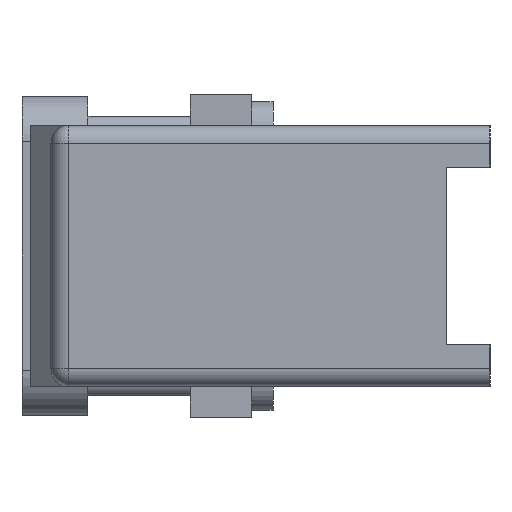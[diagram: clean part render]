
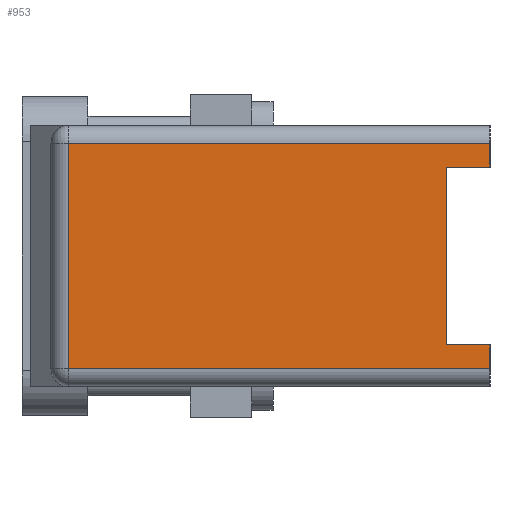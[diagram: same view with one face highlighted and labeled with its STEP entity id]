
A CAD part, left-side view. The second image highlights one B-rep face of the part: STEP entity #953.
In plain terms, the highlighted planar face has unit normal (-1, 0, 0).
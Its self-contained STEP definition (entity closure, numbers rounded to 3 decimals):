
#18 = CARTESIAN_POINT ( 'NONE',  ( 0., 3.81, -3.683 ) ) ;
#96 = CARTESIAN_POINT ( 'NONE',  ( 0., 0., -23.114 ) ) ;
#129 = CARTESIAN_POINT ( 'NONE',  ( 0., 0., -23.114 ) ) ;
#130 = VERTEX_POINT ( 'NONE', #845 ) ;
#219 = LINE ( 'NONE', #2686, #951 ) ;
#231 = LINE ( 'NONE', #2186, #2647 ) ;
#274 = LINE ( 'NONE', #713, #1966 ) ;
#310 = CARTESIAN_POINT ( 'NONE',  ( 0., 0., -23.114 ) ) ;
#330 = PLANE ( 'NONE',  #2122 ) ;
#363 = LINE ( 'NONE', #793, #1813 ) ;
#399 = EDGE_CURVE ( 'NONE', #551, #640, #274, .T. ) ;
#498 = VECTOR ( 'NONE', #2099, 1000. ) ;
#499 = VERTEX_POINT ( 'NONE', #770 ) ;
#533 = VECTOR ( 'NONE', #1638, 1000. ) ;
#551 = VERTEX_POINT ( 'NONE', #1040 ) ;
#559 = CARTESIAN_POINT ( 'NONE',  ( 0., 37.287, -23.114 ) ) ;
#625 = VERTEX_POINT ( 'NONE', #829 ) ;
#640 = VERTEX_POINT ( 'NONE', #1927 ) ;
#713 = CARTESIAN_POINT ( 'NONE',  ( 0., 3.81, -19.431 ) ) ;
#728 = VECTOR ( 'NONE', #2731, 1000. ) ;
#748 = VECTOR ( 'NONE', #1629, 1000. ) ;
#754 = EDGE_CURVE ( 'NONE', #499, #2137, #1861, .T. ) ;
#770 = CARTESIAN_POINT ( 'NONE',  ( 0., 37.287, -1.575 ) ) ;
#793 = CARTESIAN_POINT ( 'NONE',  ( 0., 3.81, -19.431 ) ) ;
#809 = DIRECTION ( 'NONE',  ( -1., 0., 0. ) ) ;
#824 = ORIENTED_EDGE ( 'NONE', *, *, #1158, .T. ) ;
#829 = CARTESIAN_POINT ( 'NONE',  ( 0., 0., -21.539 ) ) ;
#845 = CARTESIAN_POINT ( 'NONE',  ( 0., 0., -3.683 ) ) ;
#951 = VECTOR ( 'NONE', #1978, 1000. ) ;
#953 = ADVANCED_FACE ( 'NONE', ( #2273 ), #330, .T. ) ;
#964 = VERTEX_POINT ( 'NONE', #1459 ) ;
#992 = DIRECTION ( 'NONE',  ( 0., 0., 1. ) ) ;
#1039 = EDGE_CURVE ( 'NONE', #130, #2591, #1268, .T. ) ;
#1040 = CARTESIAN_POINT ( 'NONE',  ( 0., 3.81, -19.431 ) ) ;
#1124 = ORIENTED_EDGE ( 'NONE', *, *, #2693, .T. ) ;
#1140 = DIRECTION ( 'NONE',  ( 0., -1., 0. ) ) ;
#1158 = EDGE_CURVE ( 'NONE', #964, #499, #231, .T. ) ;
#1268 = LINE ( 'NONE', #1908, #498 ) ;
#1280 = DIRECTION ( 'NONE',  ( 0., 0., -1. ) ) ;
#1350 = ORIENTED_EDGE ( 'NONE', *, *, #1039, .F. ) ;
#1401 = LINE ( 'NONE', #96, #748 ) ;
#1459 = CARTESIAN_POINT ( 'NONE',  ( 0., 0., -1.575 ) ) ;
#1518 = CARTESIAN_POINT ( 'NONE',  ( 0., 37.287, -21.539 ) ) ;
#1598 = LINE ( 'NONE', #310, #533 ) ;
#1629 = DIRECTION ( 'NONE',  ( 0., 0., 1. ) ) ;
#1638 = DIRECTION ( 'NONE',  ( 0., 0., 1. ) ) ;
#1671 = ORIENTED_EDGE ( 'NONE', *, *, #754, .T. ) ;
#1691 = ORIENTED_EDGE ( 'NONE', *, *, #2351, .F. ) ;
#1813 = VECTOR ( 'NONE', #1280, 1000. ) ;
#1861 = LINE ( 'NONE', #559, #728 ) ;
#1908 = CARTESIAN_POINT ( 'NONE',  ( 0., 3.81, -3.683 ) ) ;
#1910 = ORIENTED_EDGE ( 'NONE', *, *, #2307, .T. ) ;
#1927 = CARTESIAN_POINT ( 'NONE',  ( 0., 0., -19.431 ) ) ;
#1931 = EDGE_CURVE ( 'NONE', #2137, #625, #219, .T. ) ;
#1966 = VECTOR ( 'NONE', #1140, 1000. ) ;
#1978 = DIRECTION ( 'NONE',  ( 0., -1., 0. ) ) ;
#2099 = DIRECTION ( 'NONE',  ( 0., 1., 0. ) ) ;
#2122 = AXIS2_PLACEMENT_3D ( 'NONE', #129, #809, #992 ) ;
#2137 = VERTEX_POINT ( 'NONE', #1518 ) ;
#2186 = CARTESIAN_POINT ( 'NONE',  ( 0., 38.862, -1.575 ) ) ;
#2267 = ORIENTED_EDGE ( 'NONE', *, *, #399, .F. ) ;
#2273 = FACE_OUTER_BOUND ( 'NONE', #2670, .T. ) ;
#2307 = EDGE_CURVE ( 'NONE', #130, #964, #1401, .T. ) ;
#2351 = EDGE_CURVE ( 'NONE', #2591, #551, #363, .T. ) ;
#2384 = DIRECTION ( 'NONE',  ( 0., 1., 0. ) ) ;
#2552 = ORIENTED_EDGE ( 'NONE', *, *, #1931, .T. ) ;
#2591 = VERTEX_POINT ( 'NONE', #18 ) ;
#2647 = VECTOR ( 'NONE', #2384, 1000. ) ;
#2670 = EDGE_LOOP ( 'NONE', ( #1671, #2552, #1124, #2267, #1691, #1350, #1910, #824 ) ) ;
#2686 = CARTESIAN_POINT ( 'NONE',  ( 0., 0., -21.539 ) ) ;
#2693 = EDGE_CURVE ( 'NONE', #625, #640, #1598, .T. ) ;
#2731 = DIRECTION ( 'NONE',  ( 0., 0., -1. ) ) ;
